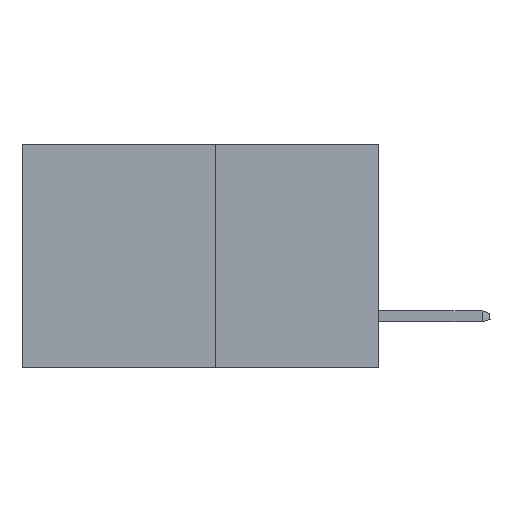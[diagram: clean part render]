
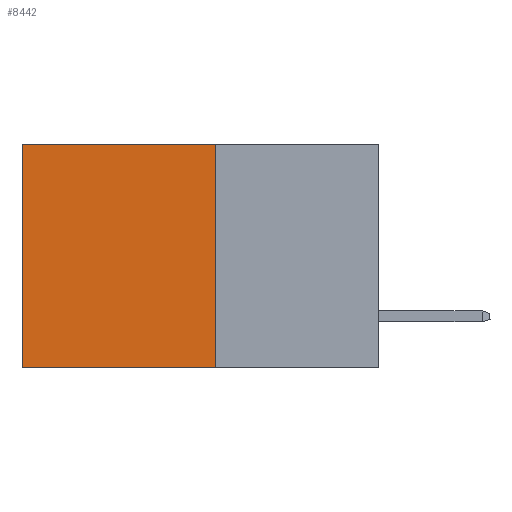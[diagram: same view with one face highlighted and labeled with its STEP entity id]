
A CAD part, left-side view. The second image highlights one B-rep face of the part: STEP entity #8442.
In plain terms, the highlighted planar face has unit normal (-1, 0, 0).
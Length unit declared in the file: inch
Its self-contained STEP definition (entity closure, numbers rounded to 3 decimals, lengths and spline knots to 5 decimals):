
#624 = VERTEX_POINT ( 'NONE', #10271 ) ;
#1196 = CARTESIAN_POINT ( 'NONE',  ( 0.277, 0.59, -0.37 ) ) ;
#1309 = CARTESIAN_POINT ( 'NONE',  ( 0.277, 0.27, -0.37 ) ) ;
#1405 = VECTOR ( 'NONE', #2487, 39.37008 ) ;
#2487 = DIRECTION ( 'NONE',  ( 0., 0., -1. ) ) ;
#2537 = CARTESIAN_POINT ( 'NONE',  ( 0.277, 0.59, -0.37 ) ) ;
#2607 = DIRECTION ( 'NONE',  ( 0., 0., -1. ) ) ;
#2660 = AXIS2_PLACEMENT_3D ( 'NONE', #1309, #10406, #2607 ) ;
#2805 = VECTOR ( 'NONE', #9132, 39.37008 ) ;
#3284 = EDGE_LOOP ( 'NONE', ( #10513, #9430, #6069, #3581 ) ) ;
#3299 = VERTEX_POINT ( 'NONE', #8528 ) ;
#3581 = ORIENTED_EDGE ( 'NONE', *, *, #8391, .T. ) ;
#3867 = EDGE_CURVE ( 'NONE', #3299, #15759, #4965, .T. ) ;
#4965 = LINE ( 'NONE', #6392, #15119 ) ;
#5037 = DIRECTION ( 'NONE',  ( 0., 1., 0. ) ) ;
#5538 = LINE ( 'NONE', #8930, #12545 ) ;
#6046 = EDGE_CURVE ( 'NONE', #9629, #3299, #13282, .T. ) ;
#6069 = ORIENTED_EDGE ( 'NONE', *, *, #6046, .F. ) ;
#6392 = CARTESIAN_POINT ( 'NONE',  ( 0.277, 0.27, -0.37 ) ) ;
#6468 = DIRECTION ( 'NONE',  ( 0., 1., 0. ) ) ;
#7773 = FACE_OUTER_BOUND ( 'NONE', #3284, .T. ) ;
#8391 = EDGE_CURVE ( 'NONE', #9629, #624, #5538, .T. ) ;
#8442 = ADVANCED_FACE ( 'NONE', ( #7773 ), #13040, .F. ) ;
#8528 = CARTESIAN_POINT ( 'NONE',  ( 0.277, 0.27, -0.37 ) ) ;
#8930 = CARTESIAN_POINT ( 'NONE',  ( 0.277, 0.27, 0. ) ) ;
#9127 = CARTESIAN_POINT ( 'NONE',  ( 0.277, 0.27, -0.37 ) ) ;
#9132 = DIRECTION ( 'NONE',  ( 0., 0., -1. ) ) ;
#9430 = ORIENTED_EDGE ( 'NONE', *, *, #3867, .F. ) ;
#9629 = VERTEX_POINT ( 'NONE', #10315 ) ;
#10271 = CARTESIAN_POINT ( 'NONE',  ( 0.277, 0.59, 0. ) ) ;
#10315 = CARTESIAN_POINT ( 'NONE',  ( 0.277, 0.27, 0. ) ) ;
#10406 = DIRECTION ( 'NONE',  ( 1., 0., 0. ) ) ;
#10513 = ORIENTED_EDGE ( 'NONE', *, *, #13748, .T. ) ;
#11828 = LINE ( 'NONE', #1196, #1405 ) ;
#12545 = VECTOR ( 'NONE', #5037, 39.37008 ) ;
#13040 = PLANE ( 'NONE',  #2660 ) ;
#13282 = LINE ( 'NONE', #9127, #2805 ) ;
#13748 = EDGE_CURVE ( 'NONE', #624, #15759, #11828, .T. ) ;
#15119 = VECTOR ( 'NONE', #6468, 39.37008 ) ;
#15759 = VERTEX_POINT ( 'NONE', #2537 ) ;
